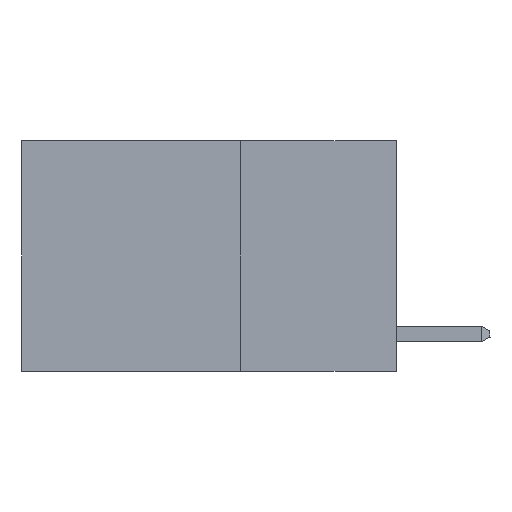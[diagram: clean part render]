
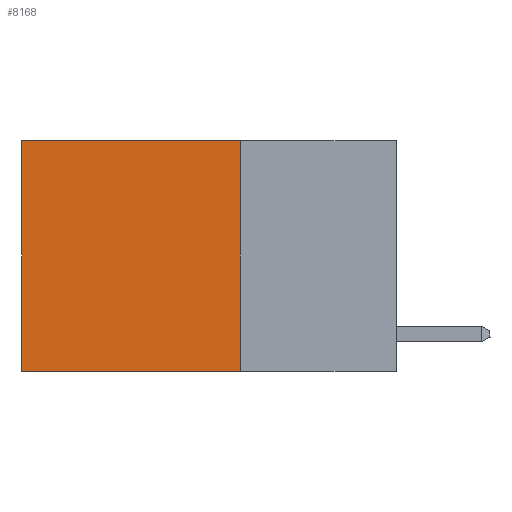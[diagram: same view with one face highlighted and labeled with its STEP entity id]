
A CAD part, left-side view. The second image highlights one B-rep face of the part: STEP entity #8168.
In plain terms, the highlighted planar face has unit normal (-1, 0, 0).
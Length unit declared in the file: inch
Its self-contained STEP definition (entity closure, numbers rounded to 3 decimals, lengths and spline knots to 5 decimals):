
#417 = CARTESIAN_POINT ( 'NONE',  ( 0.2625, 0.25, 0. ) ) ;
#455 = ORIENTED_EDGE ( 'NONE', *, *, #13295, .T. ) ;
#2624 = VERTEX_POINT ( 'NONE', #16187 ) ;
#2760 = ORIENTED_EDGE ( 'NONE', *, *, #7723, .T. ) ;
#2837 = CARTESIAN_POINT ( 'NONE',  ( 0.2625, 0.25, 0. ) ) ;
#2920 = DIRECTION ( 'NONE',  ( 0., 1., 0. ) ) ;
#3983 = DIRECTION ( 'NONE',  ( 1., 0., 0. ) ) ;
#4529 = CARTESIAN_POINT ( 'NONE',  ( 0.2625, 0.6, -0.37 ) ) ;
#5515 = VERTEX_POINT ( 'NONE', #4529 ) ;
#6052 = ORIENTED_EDGE ( 'NONE', *, *, #16339, .F. ) ;
#7002 = LINE ( 'NONE', #7781, #11559 ) ;
#7604 = CARTESIAN_POINT ( 'NONE',  ( 0.2625, 0.6, 0. ) ) ;
#7723 = EDGE_CURVE ( 'NONE', #16281, #2624, #20225, .T. ) ;
#7781 = CARTESIAN_POINT ( 'NONE',  ( 0.2625, 0.25, -0.37 ) ) ;
#8168 = ADVANCED_FACE ( 'NONE', ( #16182 ), #19450, .F. ) ;
#8590 = VECTOR ( 'NONE', #16146, 39.37008 ) ;
#10597 = EDGE_LOOP ( 'NONE', ( #455, #17500, #6052, #2760 ) ) ;
#10627 = CARTESIAN_POINT ( 'NONE',  ( 0.2625, 0.25, -0.37 ) ) ;
#10721 = EDGE_CURVE ( 'NONE', #21030, #5515, #7002, .T. ) ;
#11559 = VECTOR ( 'NONE', #19760, 39.37008 ) ;
#12513 = AXIS2_PLACEMENT_3D ( 'NONE', #417, #3983, #16067 ) ;
#13295 = EDGE_CURVE ( 'NONE', #2624, #5515, #17324, .T. ) ;
#14362 = CARTESIAN_POINT ( 'NONE',  ( 0.2625, 0.25, 0. ) ) ;
#15661 = VECTOR ( 'NONE', #2920, 39.37008 ) ;
#16067 = DIRECTION ( 'NONE',  ( 0., 0., -1. ) ) ;
#16146 = DIRECTION ( 'NONE',  ( 0., 0., -1. ) ) ;
#16182 = FACE_OUTER_BOUND ( 'NONE', #10597, .T. ) ;
#16187 = CARTESIAN_POINT ( 'NONE',  ( 0.2625, 0.6, 0. ) ) ;
#16281 = VERTEX_POINT ( 'NONE', #17645 ) ;
#16339 = EDGE_CURVE ( 'NONE', #16281, #21030, #22244, .T. ) ;
#17324 = LINE ( 'NONE', #7604, #21333 ) ;
#17500 = ORIENTED_EDGE ( 'NONE', *, *, #10721, .F. ) ;
#17645 = CARTESIAN_POINT ( 'NONE',  ( 0.2625, 0.25, 0. ) ) ;
#19450 = PLANE ( 'NONE',  #12513 ) ;
#19760 = DIRECTION ( 'NONE',  ( 0., 1., 0. ) ) ;
#20225 = LINE ( 'NONE', #2837, #15661 ) ;
#21030 = VERTEX_POINT ( 'NONE', #10627 ) ;
#21288 = DIRECTION ( 'NONE',  ( 0., 0., -1. ) ) ;
#21333 = VECTOR ( 'NONE', #21288, 39.37008 ) ;
#22244 = LINE ( 'NONE', #14362, #8590 ) ;
